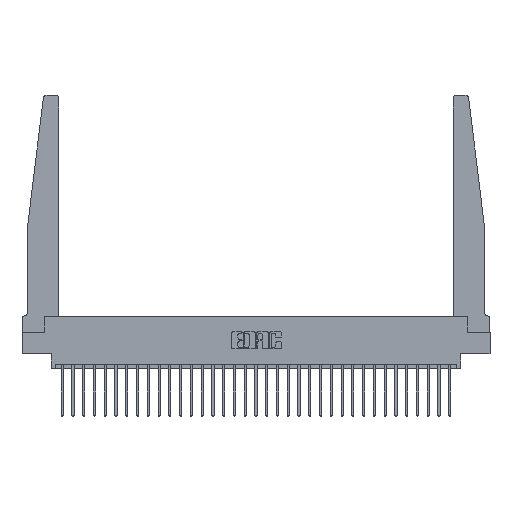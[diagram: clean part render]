
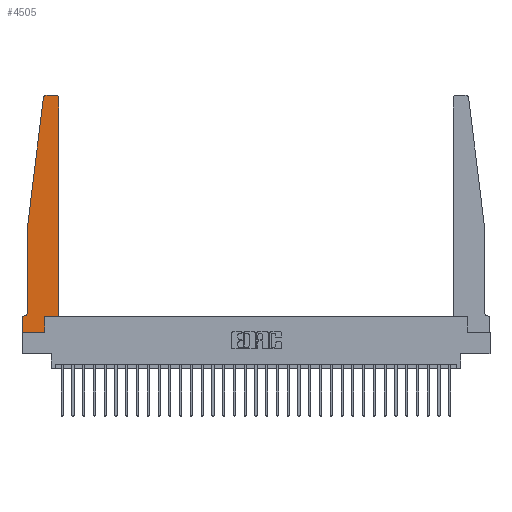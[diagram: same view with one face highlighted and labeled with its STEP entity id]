
A CAD part, top view. The second image highlights one B-rep face of the part: STEP entity #4505.
In plain terms, the highlighted planar face has unit normal (0, 0, 1).
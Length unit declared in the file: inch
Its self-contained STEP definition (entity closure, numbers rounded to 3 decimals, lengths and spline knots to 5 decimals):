
#331 = EDGE_CURVE ( 'NONE', #12492, #23202, #25404, .T. ) ;
#828 = CARTESIAN_POINT ( 'NONE',  ( 0.425, 0.18, 0.37 ) ) ;
#1790 = DIRECTION ( 'NONE',  ( -1., 0., 0. ) ) ;
#1968 = LINE ( 'NONE', #12724, #30080 ) ;
#2233 = LINE ( 'NONE', #22880, #14800 ) ;
#2372 = VERTEX_POINT ( 'NONE', #3334 ) ;
#2532 = CARTESIAN_POINT ( 'NONE',  ( 0.24675, 2.72367, 0.37 ) ) ;
#3334 = CARTESIAN_POINT ( 'NONE',  ( 0., 0.1875, 0.37 ) ) ;
#3427 = PLANE ( 'NONE',  #25505 ) ;
#3471 = CARTESIAN_POINT ( 'NONE',  ( 0.425, 2.72, 0.37 ) ) ;
#3533 = EDGE_CURVE ( 'NONE', #23202, #9312, #9782, .T. ) ;
#3562 = EDGE_CURVE ( 'NONE', #17381, #12492, #7923, .T. ) ;
#3633 = CARTESIAN_POINT ( 'NONE',  ( 0., 0., 0.37 ) ) ;
#4505 = ADVANCED_FACE ( 'NONE', ( #14911 ), #3427, .T. ) ;
#4674 = VERTEX_POINT ( 'NONE', #20998 ) ;
#5047 = CIRCLE ( 'NONE', #23597, 0.05 ) ;
#5090 = VECTOR ( 'NONE', #16838, 39.37008 ) ;
#5328 = DIRECTION ( 'NONE',  ( 0., 1., 0. ) ) ;
#5401 = EDGE_CURVE ( 'NONE', #24994, #14137, #2233, .T. ) ;
#5455 = EDGE_CURVE ( 'NONE', #26247, #20779, #5047, .T. ) ;
#6780 = CARTESIAN_POINT ( 'NONE',  ( 0., 0., 0.37 ) ) ;
#6965 = DIRECTION ( 'NONE',  ( 0., 0., -1. ) ) ;
#7209 = ORIENTED_EDGE ( 'NONE', *, *, #25799, .T. ) ;
#7225 = VERTEX_POINT ( 'NONE', #3633 ) ;
#7259 = EDGE_CURVE ( 'NONE', #2372, #7225, #25599, .T. ) ;
#7320 = CARTESIAN_POINT ( 'NONE',  ( 0.25, 2.75, 0.37 ) ) ;
#7923 = LINE ( 'NONE', #10378, #23505 ) ;
#8141 = CARTESIAN_POINT ( 'NONE',  ( 0.395, 2.75, 0.37 ) ) ;
#8271 = CARTESIAN_POINT ( 'NONE',  ( 0.395, 2.72, 0.37 ) ) ;
#8764 = DIRECTION ( 'NONE',  ( 0., 0., 1. ) ) ;
#9226 = CARTESIAN_POINT ( 'NONE',  ( 0., 0.1875, 0.37 ) ) ;
#9312 = VERTEX_POINT ( 'NONE', #16544 ) ;
#9339 = VECTOR ( 'NONE', #23380, 39.37008 ) ;
#9411 = CARTESIAN_POINT ( 'NONE',  ( 0.2605, 0., 0.37 ) ) ;
#9782 = LINE ( 'NONE', #7320, #9339 ) ;
#10021 = LINE ( 'NONE', #828, #23347 ) ;
#10378 = CARTESIAN_POINT ( 'NONE',  ( 0.425, 0.18, 0.37 ) ) ;
#10580 = CARTESIAN_POINT ( 'NONE',  ( 0.015, 0.1875, 0.37 ) ) ;
#11134 = LINE ( 'NONE', #25059, #21769 ) ;
#11873 = ORIENTED_EDGE ( 'NONE', *, *, #15482, .T. ) ;
#12229 = CARTESIAN_POINT ( 'NONE',  ( 0.065, 0.1875, 0.37 ) ) ;
#12492 = VERTEX_POINT ( 'NONE', #3471 ) ;
#12523 = DIRECTION ( 'NONE',  ( 0., 1., 0. ) ) ;
#12724 = CARTESIAN_POINT ( 'NONE',  ( 0.065, 1.25, 0.37 ) ) ;
#13008 = DIRECTION ( 'NONE',  ( 1., 0., 0. ) ) ;
#14137 = VERTEX_POINT ( 'NONE', #23796 ) ;
#14263 = CARTESIAN_POINT ( 'NONE',  ( 0.425, 0.18, 0.37 ) ) ;
#14800 = VECTOR ( 'NONE', #18146, 39.37008 ) ;
#14869 = DIRECTION ( 'NONE',  ( 1., 0., 0. ) ) ;
#14911 = FACE_OUTER_BOUND ( 'NONE', #30176, .T. ) ;
#15418 = ORIENTED_EDGE ( 'NONE', *, *, #5455, .T. ) ;
#15482 = EDGE_CURVE ( 'NONE', #29273, #4674, #19707, .T. ) ;
#16544 = CARTESIAN_POINT ( 'NONE',  ( 0.27653, 2.75, 0.37 ) ) ;
#16838 = DIRECTION ( 'NONE',  ( -1., 0., 0. ) ) ;
#17381 = VERTEX_POINT ( 'NONE', #14263 ) ;
#17943 = EDGE_CURVE ( 'NONE', #20779, #2372, #21276, .T. ) ;
#18146 = DIRECTION ( 'NONE',  ( -0.122, -0.992, 0. ) ) ;
#18758 = CARTESIAN_POINT ( 'NONE',  ( 0.015, 0.2375, 0.37 ) ) ;
#19488 = EDGE_CURVE ( 'NONE', #7225, #29273, #11134, .T. ) ;
#19707 = LINE ( 'NONE', #24434, #28421 ) ;
#19942 = AXIS2_PLACEMENT_3D ( 'NONE', #24481, #29057, #13008 ) ;
#20459 = ORIENTED_EDGE ( 'NONE', *, *, #5401, .T. ) ;
#20779 = VERTEX_POINT ( 'NONE', #10580 ) ;
#20863 = DIRECTION ( 'NONE',  ( 0., -1., 0. ) ) ;
#20976 = ORIENTED_EDGE ( 'NONE', *, *, #3562, .T. ) ;
#20998 = CARTESIAN_POINT ( 'NONE',  ( 0.2605, 0.18, 0.37 ) ) ;
#21276 = LINE ( 'NONE', #12229, #5090 ) ;
#21769 = VECTOR ( 'NONE', #30083, 39.37008 ) ;
#22690 = DIRECTION ( 'NONE',  ( 1., 0., 0. ) ) ;
#22880 = CARTESIAN_POINT ( 'NONE',  ( 0.065, 1.25, 0.37 ) ) ;
#23034 = CARTESIAN_POINT ( 'NONE',  ( 0.065, 0.2375, 0.37 ) ) ;
#23138 = ORIENTED_EDGE ( 'NONE', *, *, #3533, .T. ) ;
#23202 = VERTEX_POINT ( 'NONE', #8141 ) ;
#23347 = VECTOR ( 'NONE', #28646, 39.37008 ) ;
#23380 = DIRECTION ( 'NONE',  ( -1., 0., 0. ) ) ;
#23505 = VECTOR ( 'NONE', #5328, 39.37008 ) ;
#23597 = AXIS2_PLACEMENT_3D ( 'NONE', #18758, #6965, #1790 ) ;
#23796 = CARTESIAN_POINT ( 'NONE',  ( 0.065, 1.25, 0.37 ) ) ;
#24347 = CIRCLE ( 'NONE', #19942, 0.03 ) ;
#24434 = CARTESIAN_POINT ( 'NONE',  ( 0.2605, 0.18, 0.37 ) ) ;
#24481 = CARTESIAN_POINT ( 'NONE',  ( 0.27653, 2.72, 0.37 ) ) ;
#24994 = VERTEX_POINT ( 'NONE', #2532 ) ;
#25059 = CARTESIAN_POINT ( 'NONE',  ( 0., 0., 0.37 ) ) ;
#25404 = CIRCLE ( 'NONE', #28312, 0.03 ) ;
#25505 = AXIS2_PLACEMENT_3D ( 'NONE', #9226, #8764, #22690 ) ;
#25599 = LINE ( 'NONE', #6780, #27407 ) ;
#25799 = EDGE_CURVE ( 'NONE', #14137, #26247, #1968, .T. ) ;
#26247 = VERTEX_POINT ( 'NONE', #23034 ) ;
#26730 = ORIENTED_EDGE ( 'NONE', *, *, #7259, .T. ) ;
#27190 = ORIENTED_EDGE ( 'NONE', *, *, #29411, .T. ) ;
#27407 = VECTOR ( 'NONE', #20863, 39.37008 ) ;
#28273 = ORIENTED_EDGE ( 'NONE', *, *, #19488, .T. ) ;
#28312 = AXIS2_PLACEMENT_3D ( 'NONE', #8271, #29061, #14869 ) ;
#28421 = VECTOR ( 'NONE', #12523, 39.37008 ) ;
#28646 = DIRECTION ( 'NONE',  ( 1., 0., 0. ) ) ;
#29028 = ORIENTED_EDGE ( 'NONE', *, *, #331, .T. ) ;
#29057 = DIRECTION ( 'NONE',  ( 0., 0., 1. ) ) ;
#29061 = DIRECTION ( 'NONE',  ( 0., 0., 1. ) ) ;
#29068 = DIRECTION ( 'NONE',  ( 0., -1., 0. ) ) ;
#29195 = ORIENTED_EDGE ( 'NONE', *, *, #17943, .T. ) ;
#29273 = VERTEX_POINT ( 'NONE', #9411 ) ;
#29411 = EDGE_CURVE ( 'NONE', #4674, #17381, #10021, .T. ) ;
#29832 = EDGE_CURVE ( 'NONE', #9312, #24994, #24347, .T. ) ;
#29881 = ORIENTED_EDGE ( 'NONE', *, *, #29832, .T. ) ;
#30080 = VECTOR ( 'NONE', #29068, 39.37008 ) ;
#30083 = DIRECTION ( 'NONE',  ( 1., 0., 0. ) ) ;
#30176 = EDGE_LOOP ( 'NONE', ( #23138, #29881, #20459, #7209, #15418, #29195, #26730, #28273, #11873, #27190, #20976, #29028 ) ) ;
